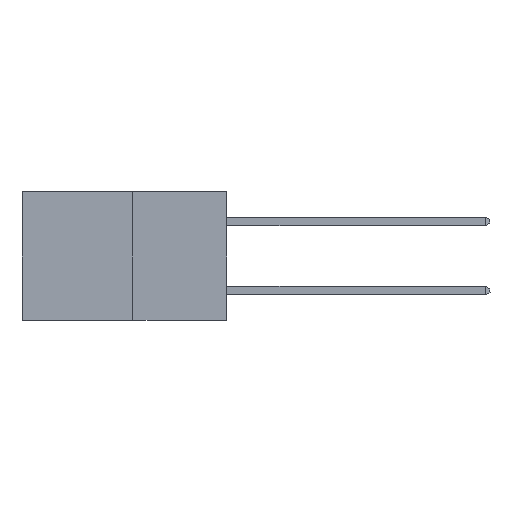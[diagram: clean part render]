
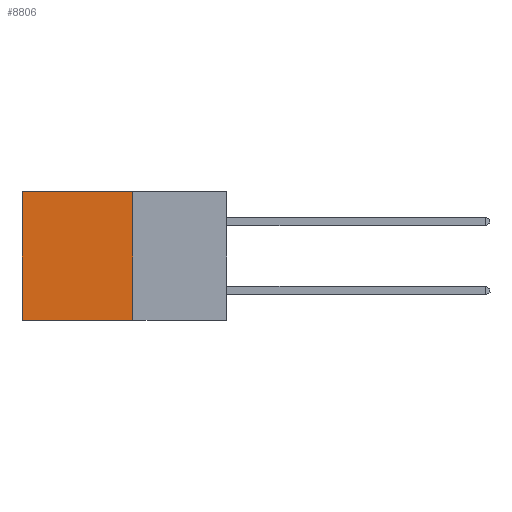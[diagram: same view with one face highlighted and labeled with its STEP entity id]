
A CAD part, left-side view. The second image highlights one B-rep face of the part: STEP entity #8806.
In plain terms, the highlighted planar face has unit normal (-1, 0, 0).
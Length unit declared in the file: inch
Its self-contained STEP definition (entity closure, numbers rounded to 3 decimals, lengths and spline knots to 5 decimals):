
#1284 = CARTESIAN_POINT ( 'NONE',  ( 0.277, 0.59, 0. ) ) ;
#1368 = EDGE_CURVE ( 'NONE', #16693, #2047, #26529, .T. ) ;
#1558 = VERTEX_POINT ( 'NONE', #6862 ) ;
#2047 = VERTEX_POINT ( 'NONE', #26367 ) ;
#2595 = CARTESIAN_POINT ( 'NONE',  ( 0.277, 0.27, -0.37 ) ) ;
#2671 = DIRECTION ( 'NONE',  ( 0., 0., -1. ) ) ;
#3311 = CARTESIAN_POINT ( 'NONE',  ( 0.277, 0.27, -0.37 ) ) ;
#4078 = EDGE_CURVE ( 'NONE', #1558, #29625, #28561, .T. ) ;
#4778 = LINE ( 'NONE', #3311, #16830 ) ;
#5550 = ORIENTED_EDGE ( 'NONE', *, *, #11932, .F. ) ;
#5734 = DIRECTION ( 'NONE',  ( 0., 0., -1. ) ) ;
#6862 = CARTESIAN_POINT ( 'NONE',  ( 0.277, 0.27, 0. ) ) ;
#8806 = ADVANCED_FACE ( 'NONE', ( #19954 ), #12321, .F. ) ;
#8887 = EDGE_CURVE ( 'NONE', #29625, #2047, #23274, .T. ) ;
#11932 = EDGE_CURVE ( 'NONE', #1558, #16693, #4778, .T. ) ;
#12321 = PLANE ( 'NONE',  #24894 ) ;
#12731 = CARTESIAN_POINT ( 'NONE',  ( 0.277, 0.27, 0. ) ) ;
#13324 = DIRECTION ( 'NONE',  ( 0., 1., 0. ) ) ;
#14451 = ORIENTED_EDGE ( 'NONE', *, *, #4078, .T. ) ;
#16021 = VECTOR ( 'NONE', #13324, 39.37008 ) ;
#16693 = VERTEX_POINT ( 'NONE', #26214 ) ;
#16830 = VECTOR ( 'NONE', #5734, 39.37008 ) ;
#16971 = VECTOR ( 'NONE', #17409, 39.37008 ) ;
#17097 = DIRECTION ( 'NONE',  ( 1., 0., 0. ) ) ;
#17409 = DIRECTION ( 'NONE',  ( 0., 0., -1. ) ) ;
#18777 = VECTOR ( 'NONE', #30530, 39.37008 ) ;
#19954 = FACE_OUTER_BOUND ( 'NONE', #25282, .T. ) ;
#20537 = ORIENTED_EDGE ( 'NONE', *, *, #8887, .T. ) ;
#21759 = CARTESIAN_POINT ( 'NONE',  ( 0.277, 0.27, -0.37 ) ) ;
#23274 = LINE ( 'NONE', #24451, #16971 ) ;
#24391 = ORIENTED_EDGE ( 'NONE', *, *, #1368, .F. ) ;
#24451 = CARTESIAN_POINT ( 'NONE',  ( 0.277, 0.59, -0.37 ) ) ;
#24894 = AXIS2_PLACEMENT_3D ( 'NONE', #21759, #17097, #2671 ) ;
#25282 = EDGE_LOOP ( 'NONE', ( #20537, #24391, #5550, #14451 ) ) ;
#26214 = CARTESIAN_POINT ( 'NONE',  ( 0.277, 0.27, -0.37 ) ) ;
#26367 = CARTESIAN_POINT ( 'NONE',  ( 0.277, 0.59, -0.37 ) ) ;
#26529 = LINE ( 'NONE', #2595, #18777 ) ;
#28561 = LINE ( 'NONE', #12731, #16021 ) ;
#29625 = VERTEX_POINT ( 'NONE', #1284 ) ;
#30530 = DIRECTION ( 'NONE',  ( 0., 1., 0. ) ) ;
